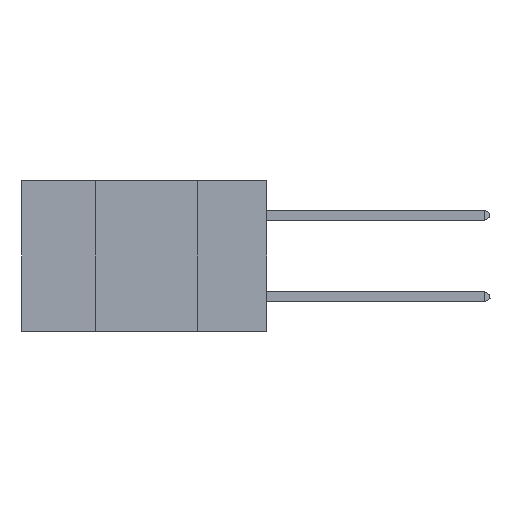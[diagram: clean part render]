
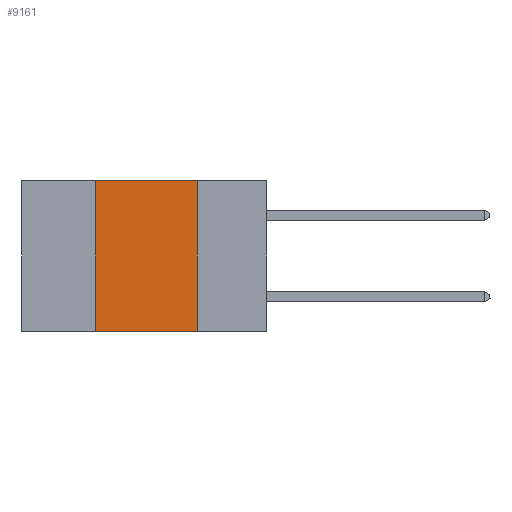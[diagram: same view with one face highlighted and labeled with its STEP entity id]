
A CAD part, left-side view. The second image highlights one B-rep face of the part: STEP entity #9161.
In plain terms, the highlighted planar face has unit normal (-1, 0, 0).
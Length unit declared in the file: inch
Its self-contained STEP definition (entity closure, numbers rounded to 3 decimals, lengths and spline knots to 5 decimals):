
#440 = VECTOR ( 'NONE', #13027, 39.37008 ) ;
#2326 = EDGE_CURVE ( 'NONE', #23258, #3504, #4134, .T. ) ;
#3409 = CARTESIAN_POINT ( 'NONE',  ( 0., 0.17, 0. ) ) ;
#3504 = VERTEX_POINT ( 'NONE', #19229 ) ;
#4134 = LINE ( 'NONE', #11521, #440 ) ;
#5926 = LINE ( 'NONE', #20827, #14626 ) ;
#6513 = EDGE_CURVE ( 'NONE', #26808, #11988, #15805, .T. ) ;
#7213 = PLANE ( 'NONE',  #21393 ) ;
#7543 = EDGE_CURVE ( 'NONE', #3504, #26808, #8338, .T. ) ;
#7920 = DIRECTION ( 'NONE',  ( 0., -1., 0. ) ) ;
#8338 = LINE ( 'NONE', #13296, #17072 ) ;
#9161 = ADVANCED_FACE ( 'NONE', ( #17675 ), #7213, .F. ) ;
#9524 = EDGE_CURVE ( 'NONE', #23258, #11988, #5926, .T. ) ;
#9938 = DIRECTION ( 'NONE',  ( 0., 0., -1. ) ) ;
#10728 = ORIENTED_EDGE ( 'NONE', *, *, #6513, .F. ) ;
#11521 = CARTESIAN_POINT ( 'NONE',  ( 0., 0.42, 0. ) ) ;
#11988 = VERTEX_POINT ( 'NONE', #19468 ) ;
#12814 = ORIENTED_EDGE ( 'NONE', *, *, #2326, .F. ) ;
#13027 = DIRECTION ( 'NONE',  ( 0., 0., 1. ) ) ;
#13296 = CARTESIAN_POINT ( 'NONE',  ( 0., 0.6, 0. ) ) ;
#14218 = DIRECTION ( 'NONE',  ( 0., -1., 0. ) ) ;
#14626 = VECTOR ( 'NONE', #7920, 39.37008 ) ;
#15805 = LINE ( 'NONE', #3409, #19181 ) ;
#17072 = VECTOR ( 'NONE', #14218, 39.37008 ) ;
#17675 = FACE_OUTER_BOUND ( 'NONE', #26201, .T. ) ;
#17921 = CARTESIAN_POINT ( 'NONE',  ( 0., 0.6, 0. ) ) ;
#18910 = CARTESIAN_POINT ( 'NONE',  ( 0., 0.17, 0. ) ) ;
#19181 = VECTOR ( 'NONE', #9938, 39.37008 ) ;
#19229 = CARTESIAN_POINT ( 'NONE',  ( 0., 0.42, 0. ) ) ;
#19468 = CARTESIAN_POINT ( 'NONE',  ( 0., 0.17, -0.37 ) ) ;
#20827 = CARTESIAN_POINT ( 'NONE',  ( 0., 0.6, -0.37 ) ) ;
#20927 = CARTESIAN_POINT ( 'NONE',  ( 0., 0.42, -0.37 ) ) ;
#21393 = AXIS2_PLACEMENT_3D ( 'NONE', #17921, #24388, #24585 ) ;
#23258 = VERTEX_POINT ( 'NONE', #20927 ) ;
#24388 = DIRECTION ( 'NONE',  ( 1., 0., 0. ) ) ;
#24585 = DIRECTION ( 'NONE',  ( 0., 0., -1. ) ) ;
#24586 = ORIENTED_EDGE ( 'NONE', *, *, #7543, .F. ) ;
#25309 = ORIENTED_EDGE ( 'NONE', *, *, #9524, .T. ) ;
#26201 = EDGE_LOOP ( 'NONE', ( #10728, #24586, #12814, #25309 ) ) ;
#26808 = VERTEX_POINT ( 'NONE', #18910 ) ;
